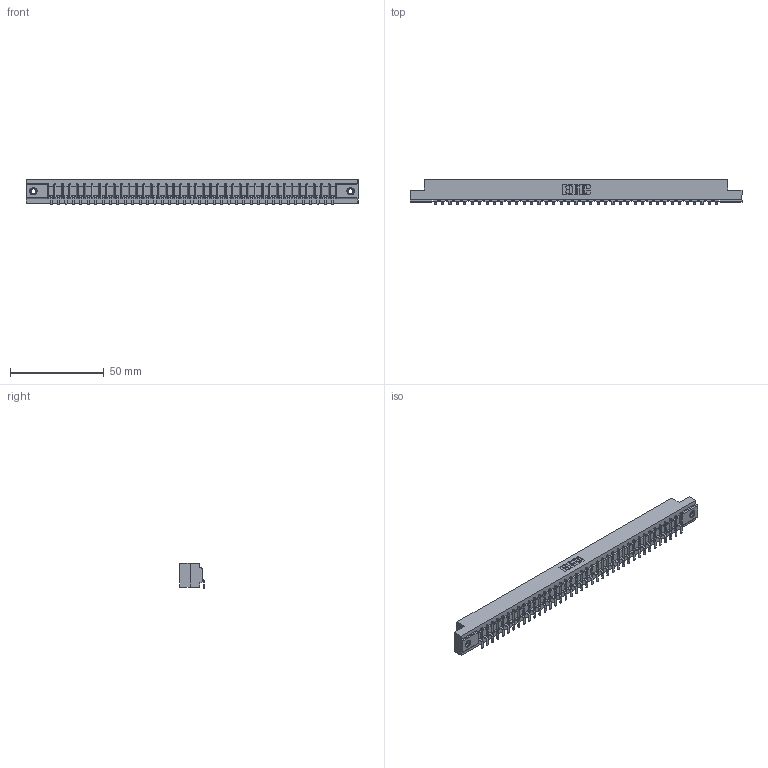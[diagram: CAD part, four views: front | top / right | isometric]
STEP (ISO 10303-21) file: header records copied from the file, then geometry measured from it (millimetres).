
FILE_DESCRIPTION (( 'STEP AP203' ), '1' );
FILE_NAME ('307-039-453-107.STEP', '2020-09-29T08:36:15', ( '' ), ( '' ), 'SwSTEP 2.0', 'SolidWorks 2020', '' );
FILE_SCHEMA (( 'CONFIG_CONTROL_DESIGN' ));
Length unit declared in the file: inch
Products named in the file (4): 345-250-001_345-250-005-103; 307 Part_.156 Dia Mounting Holes; 307-290-002_553; 307-039-453-107
Assembly tree (42 placements, depth 2):
  307-039-453-107
    307 Part_.156 Dia Mounting Holes
    307-290-002_553  x39
    345-250-001_345-250-005-103  x2
Bounding box: 177.55 x 13.32 x 13.5 mm (x, y, z)
Volume: 18963.6 mm3; surface area: 23804.4 mm2
Topology: 42 solids, 42 shells, 3260 faces, 9975 edges, 6534 vertices
Faces by surface type: plane 1935, cylinder 1229, sphere 80, cone 12, torus 4
Entity records: 35843 total; most frequent: CARTESIAN_POINT 6027, ORIENTED_EDGE 6010, DIRECTION 5867, EDGE_CURVE 3005, VECTOR 2299, LINE 2299, VERTEX_POINT 1944, AXIS2_PLACEMENT_3D 1784
